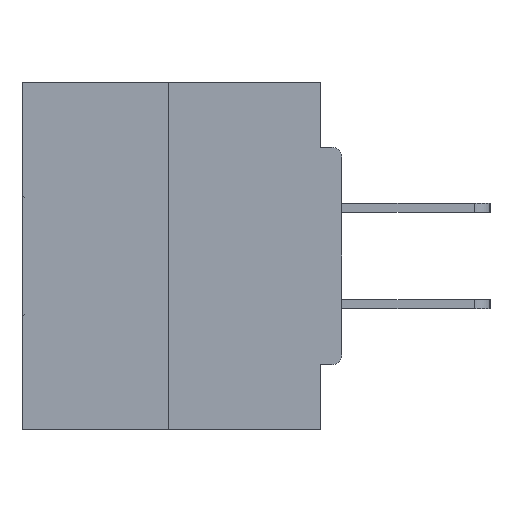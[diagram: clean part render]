
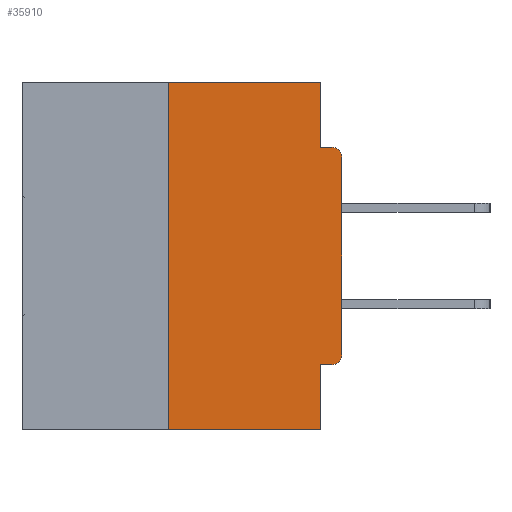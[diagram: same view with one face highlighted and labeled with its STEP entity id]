
A CAD part, left-side view. The second image highlights one B-rep face of the part: STEP entity #35910.
In plain terms, the highlighted planar face has unit normal (-1, 0, 0).
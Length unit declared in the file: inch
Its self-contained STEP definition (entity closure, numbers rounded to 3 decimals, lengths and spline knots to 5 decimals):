
#594 = LINE ( 'NONE', #6286, #35868 ) ;
#1430 = CARTESIAN_POINT ( 'NONE',  ( 0., 0.015, -0.1085 ) ) ;
#1570 = DIRECTION ( 'NONE',  ( -1., 0., 0. ) ) ;
#1732 = CARTESIAN_POINT ( 'NONE',  ( 0., 0.46, 0. ) ) ;
#2965 = LINE ( 'NONE', #23147, #28901 ) ;
#5306 = DIRECTION ( 'NONE',  ( -1., 0., 0. ) ) ;
#5801 = ORIENTED_EDGE ( 'NONE', *, *, #36532, .F. ) ;
#6286 = CARTESIAN_POINT ( 'NONE',  ( 0., 0.25, 0. ) ) ;
#7032 = CARTESIAN_POINT ( 'NONE',  ( 0., 0.015, -0.4065 ) ) ;
#7473 = LINE ( 'NONE', #1732, #36788 ) ;
#7753 = DIRECTION ( 'NONE',  ( 0., 0., -1. ) ) ;
#8060 = DIRECTION ( 'NONE',  ( 0., -1., 0. ) ) ;
#8579 = CIRCLE ( 'NONE', #22383, 0.015 ) ;
#9908 = ORIENTED_EDGE ( 'NONE', *, *, #30273, .F. ) ;
#11244 = VECTOR ( 'NONE', #38850, 39.37008 ) ;
#11332 = CARTESIAN_POINT ( 'NONE',  ( 0., 0.015, -0.3915 ) ) ;
#11809 = ORIENTED_EDGE ( 'NONE', *, *, #35991, .T. ) ;
#12100 = VECTOR ( 'NONE', #25854, 39.37008 ) ;
#13747 = EDGE_LOOP ( 'NONE', ( #31251, #24770, #17021, #5801, #26064, #11809, #23459, #27169, #9908, #37000 ) ) ;
#14111 = VERTEX_POINT ( 'NONE', #24630 ) ;
#14248 = EDGE_CURVE ( 'NONE', #21750, #26141, #31778, .T. ) ;
#14352 = EDGE_CURVE ( 'NONE', #17092, #37811, #15627, .T. ) ;
#15360 = CARTESIAN_POINT ( 'NONE',  ( 0., 0., -0.3915 ) ) ;
#15537 = EDGE_CURVE ( 'NONE', #28875, #32835, #32149, .T. ) ;
#15627 = LINE ( 'NONE', #39116, #39143 ) ;
#15817 = LINE ( 'NONE', #26443, #20757 ) ;
#16739 = CARTESIAN_POINT ( 'NONE',  ( 0., 0., -0.0935 ) ) ;
#17021 = ORIENTED_EDGE ( 'NONE', *, *, #40453, .T. ) ;
#17092 = VERTEX_POINT ( 'NONE', #7032 ) ;
#17662 = AXIS2_PLACEMENT_3D ( 'NONE', #39358, #26769, #30313 ) ;
#18363 = EDGE_CURVE ( 'NONE', #26141, #31250, #35352, .T. ) ;
#20115 = CARTESIAN_POINT ( 'NONE',  ( 0., 0., 0. ) ) ;
#20399 = DIRECTION ( 'NONE',  ( 0., 1., 0. ) ) ;
#20521 = DIRECTION ( 'NONE',  ( 0., 0., -1. ) ) ;
#20757 = VECTOR ( 'NONE', #7753, 39.37008 ) ;
#21371 = CARTESIAN_POINT ( 'NONE',  ( 0., 0.031, -0.4065 ) ) ;
#21458 = CARTESIAN_POINT ( 'NONE',  ( 0., 0.031, -0.0935 ) ) ;
#21750 = VERTEX_POINT ( 'NONE', #15360 ) ;
#22383 = AXIS2_PLACEMENT_3D ( 'NONE', #11332, #5306, #20521 ) ;
#23147 = CARTESIAN_POINT ( 'NONE',  ( 0., 0.46, -0.5 ) ) ;
#23459 = ORIENTED_EDGE ( 'NONE', *, *, #14248, .T. ) ;
#23479 = VERTEX_POINT ( 'NONE', #29937 ) ;
#23910 = CARTESIAN_POINT ( 'NONE',  ( 0., 0.015, -0.0935 ) ) ;
#24630 = CARTESIAN_POINT ( 'NONE',  ( 0., 0.25, -0.5 ) ) ;
#24770 = ORIENTED_EDGE ( 'NONE', *, *, #38858, .F. ) ;
#25854 = DIRECTION ( 'NONE',  ( 0., 0., -1. ) ) ;
#26064 = ORIENTED_EDGE ( 'NONE', *, *, #14352, .F. ) ;
#26141 = VERTEX_POINT ( 'NONE', #28271 ) ;
#26443 = CARTESIAN_POINT ( 'NONE',  ( 0., 0.031, -0.5 ) ) ;
#26769 = DIRECTION ( 'NONE',  ( 1., 0., 0. ) ) ;
#27021 = CARTESIAN_POINT ( 'NONE',  ( 0., 0.25, 0. ) ) ;
#27169 = ORIENTED_EDGE ( 'NONE', *, *, #18363, .T. ) ;
#28142 = DIRECTION ( 'NONE',  ( 0., 0., 1. ) ) ;
#28271 = CARTESIAN_POINT ( 'NONE',  ( 0., 0., -0.1085 ) ) ;
#28875 = VERTEX_POINT ( 'NONE', #35350 ) ;
#28901 = VECTOR ( 'NONE', #32283, 39.37008 ) ;
#29937 = CARTESIAN_POINT ( 'NONE',  ( 0., 0.031, -0.5 ) ) ;
#30273 = EDGE_CURVE ( 'NONE', #32835, #31250, #32053, .T. ) ;
#30313 = DIRECTION ( 'NONE',  ( 0., 0., -1. ) ) ;
#30574 = VECTOR ( 'NONE', #38628, 39.37008 ) ;
#31213 = VERTEX_POINT ( 'NONE', #27021 ) ;
#31250 = VERTEX_POINT ( 'NONE', #23910 ) ;
#31251 = ORIENTED_EDGE ( 'NONE', *, *, #39140, .F. ) ;
#31537 = FACE_OUTER_BOUND ( 'NONE', #13747, .T. ) ;
#31778 = LINE ( 'NONE', #20115, #11244 ) ;
#32053 = LINE ( 'NONE', #16739, #30574 ) ;
#32149 = LINE ( 'NONE', #35581, #12100 ) ;
#32283 = DIRECTION ( 'NONE',  ( 0., -1., 0. ) ) ;
#32835 = VERTEX_POINT ( 'NONE', #21458 ) ;
#35350 = CARTESIAN_POINT ( 'NONE',  ( 0., 0.031, 0. ) ) ;
#35352 = CIRCLE ( 'NONE', #36931, 0.015 ) ;
#35581 = CARTESIAN_POINT ( 'NONE',  ( 0., 0.031, 0. ) ) ;
#35868 = VECTOR ( 'NONE', #28142, 39.37008 ) ;
#35910 = ADVANCED_FACE ( 'NONE', ( #31537 ), #39500, .F. ) ;
#35991 = EDGE_CURVE ( 'NONE', #17092, #21750, #8579, .T. ) ;
#36532 = EDGE_CURVE ( 'NONE', #37811, #23479, #15817, .T. ) ;
#36788 = VECTOR ( 'NONE', #8060, 39.37008 ) ;
#36931 = AXIS2_PLACEMENT_3D ( 'NONE', #1430, #1570, #38939 ) ;
#37000 = ORIENTED_EDGE ( 'NONE', *, *, #15537, .F. ) ;
#37811 = VERTEX_POINT ( 'NONE', #21371 ) ;
#38628 = DIRECTION ( 'NONE',  ( 0., -1., 0. ) ) ;
#38850 = DIRECTION ( 'NONE',  ( 0., 0., 1. ) ) ;
#38858 = EDGE_CURVE ( 'NONE', #14111, #31213, #594, .T. ) ;
#38939 = DIRECTION ( 'NONE',  ( 0., 0., -1. ) ) ;
#39116 = CARTESIAN_POINT ( 'NONE',  ( 0., 0., -0.4065 ) ) ;
#39140 = EDGE_CURVE ( 'NONE', #31213, #28875, #7473, .T. ) ;
#39143 = VECTOR ( 'NONE', #20399, 39.37008 ) ;
#39358 = CARTESIAN_POINT ( 'NONE',  ( 0., 0.46, 0. ) ) ;
#39500 = PLANE ( 'NONE',  #17662 ) ;
#40453 = EDGE_CURVE ( 'NONE', #14111, #23479, #2965, .T. ) ;
